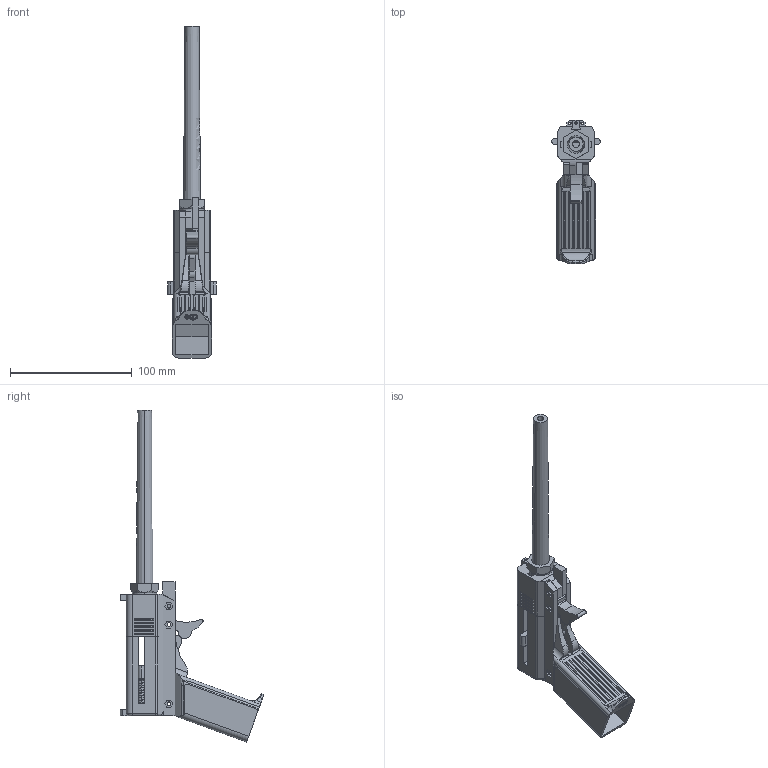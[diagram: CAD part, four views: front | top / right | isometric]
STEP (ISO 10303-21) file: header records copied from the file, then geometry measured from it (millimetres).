
FILE_DESCRIPTION (( 'STEP AP214' ), '1' );
FILE_NAME ('StikM1.STEP', '2013-09-01T22:29:57', ( 'Asher' ), ( '' ), 'SwSTEP 2.0', 'SolidWorks 2013', '' );
FILE_SCHEMA (( 'AUTOMOTIVE_DESIGN' ));
Length unit declared in the file: millimetre
Products named in the file (14): RearSight^StikM1; LowerGrip^StikM1; SpringComp^StikM1; FrontSight^StikM1; Bolt^StikM1; UpperFrame^StikM1; Receiver^StikM1; BarrelAndChamber; StikM1; TriggerGuard^StikM1; SearPin^StikM1; Barrel^StikM1; Trigger; Sear
Assembly tree (13 placements, depth 2):
  StikM1
    BarrelAndChamber
    Receiver^StikM1
    UpperFrame^StikM1
    Bolt^StikM1
    FrontSight^StikM1
    SpringComp^StikM1
    LowerGrip^StikM1
    RearSight^StikM1
    Sear
    Trigger
    Barrel^StikM1
    SearPin^StikM1
    TriggerGuard^StikM1
Bounding box: 40 x 117.88 x 272.38 mm (x, y, z)
Volume: 143310.1 mm3; surface area: 68072.7 mm2
Topology: 13 solids, 13 shells, 1173 faces, 3240 edges, 2134 vertices
Faces by surface type: plane 547, bspline 343, cylinder 251, cone 28, torus 4
Entity records: 58382 total; most frequent: CARTESIAN_POINT 30594, ORIENTED_EDGE 6472, DIRECTION 4358, EDGE_CURVE 3236, VERTEX_POINT 2134, LINE 1844, VECTOR 1844, EDGE_LOOP 1262
